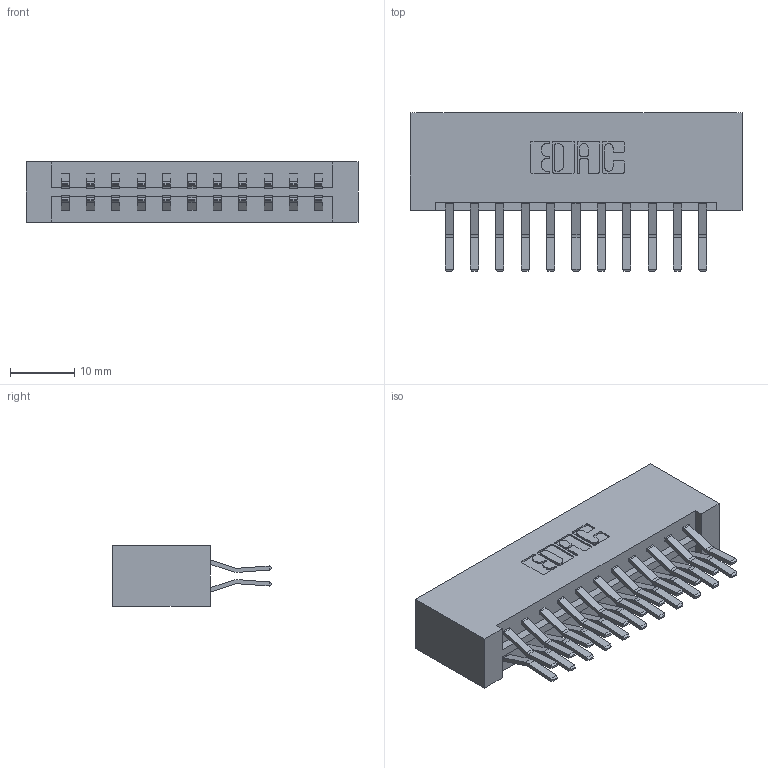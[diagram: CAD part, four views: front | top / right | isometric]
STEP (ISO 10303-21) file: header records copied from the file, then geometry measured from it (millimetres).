
FILE_DESCRIPTION (( 'STEP AP203' ), '1' );
FILE_NAME ('833-022-560-201.STEP', '2020-06-01T18:25:57', ( '' ), ( '' ), 'SwSTEP 2.0', 'SolidWorks 2020', '' );
FILE_SCHEMA (( 'CONFIG_CONTROL_DESIGN' ));
Length unit declared in the file: inch
Products named in the file (3): 833-022-560-201; 833 Part_Lugless; 345-292-001_560 Tail
Assembly tree (23 placements, depth 2):
  833-022-560-201
    833 Part_Lugless
    345-292-001_560 Tail  x22
Bounding box: 51.84 x 24.78 x 9.4 mm (x, y, z)
Volume: 5779.2 mm3; surface area: 6935.1 mm2
Topology: 23 solids, 23 shells, 1294 faces, 3829 edges, 2522 vertices
Faces by surface type: plane 858, cylinder 436
Entity records: 10897 total; most frequent: CARTESIAN_POINT 1842, ORIENTED_EDGE 1778, DIRECTION 1625, EDGE_CURVE 889, VECTOR 765, LINE 765, VERTEX_POINT 590, AXIS2_PLACEMENT_3D 430
